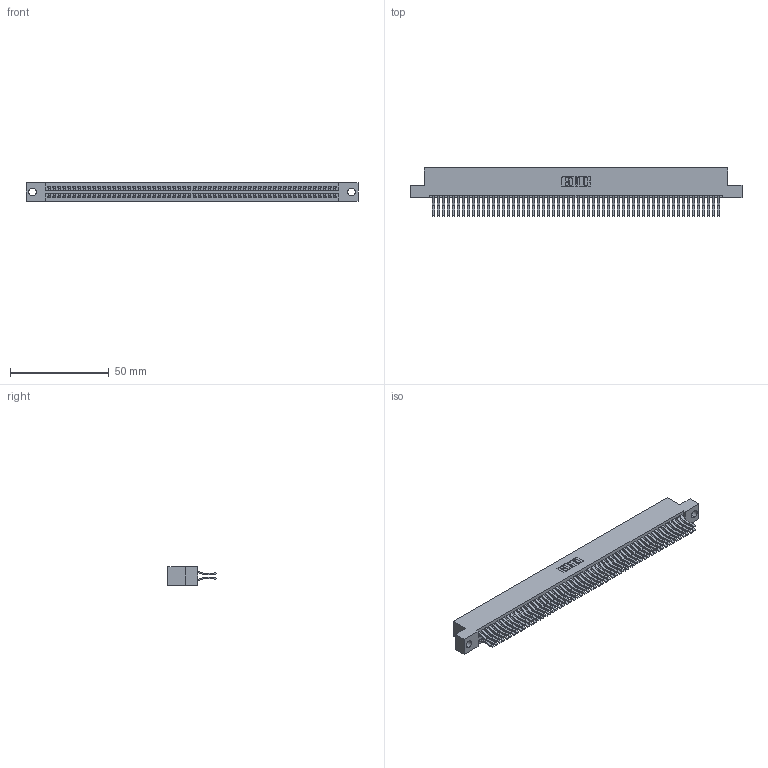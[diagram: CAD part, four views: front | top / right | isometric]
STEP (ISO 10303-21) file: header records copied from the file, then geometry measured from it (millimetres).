
FILE_DESCRIPTION (( 'STEP AP203' ), '1' );
FILE_NAME ('345-116-560-204.STEP', '2018-10-18T20:29:21', ( '' ), ( '' ), 'SwSTEP 2.0', 'SolidWorks 2016', '' );
FILE_SCHEMA (( 'CONFIG_CONTROL_DESIGN' ));
Length unit declared in the file: inch
Products named in the file (3): 345-292-001_560 Tail; 345 Part_Flush Mounting Lugs - 0.156 Dia-TH; 345-116-560-204
Assembly tree (117 placements, depth 2):
  345-116-560-204
    345 Part_Flush Mounting Lugs - 0.156 Dia-TH
    345-292-001_560 Tail  x116
Bounding box: 168.53 x 24.45 x 9.4 mm (x, y, z)
Volume: 17192.1 mm3; surface area: 27493.3 mm2
Topology: 117 solids, 117 shells, 6158 faces, 18321 edges, 12058 vertices
Faces by surface type: plane 3908, cylinder 2250
Entity records: 43445 total; most frequent: CARTESIAN_POINT 7268, ORIENTED_EDGE 7202, DIRECTION 6393, EDGE_CURVE 3601, LINE 3233, VECTOR 3233, VERTEX_POINT 2398, AXIS2_PLACEMENT_3D 1580
